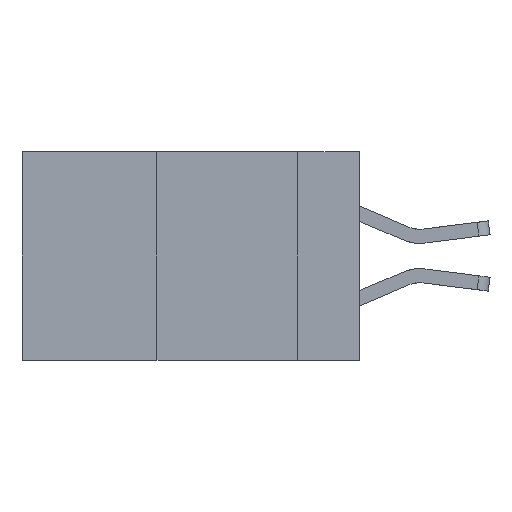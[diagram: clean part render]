
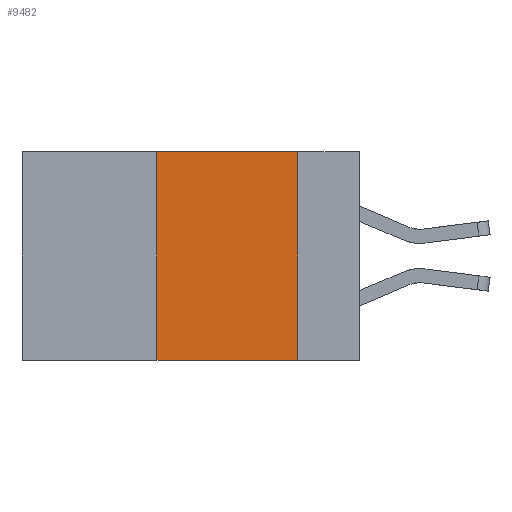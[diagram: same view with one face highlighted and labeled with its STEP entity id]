
A CAD part, left-side view. The second image highlights one B-rep face of the part: STEP entity #9482.
In plain terms, the highlighted planar face has unit normal (-1, 0, 0).
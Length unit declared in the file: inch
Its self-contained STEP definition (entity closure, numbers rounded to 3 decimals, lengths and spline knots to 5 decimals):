
#306 = EDGE_CURVE ( 'NONE', #2937, #2460, #10164, .T. ) ;
#478 = VECTOR ( 'NONE', #8379, 39.37008 ) ;
#971 = LINE ( 'NONE', #3091, #1587 ) ;
#1077 = VECTOR ( 'NONE', #9889, 39.37008 ) ;
#1249 = ORIENTED_EDGE ( 'NONE', *, *, #306, .T. ) ;
#1296 = CARTESIAN_POINT ( 'NONE',  ( 0., 0.11, -0.37 ) ) ;
#1587 = VECTOR ( 'NONE', #3090, 39.37008 ) ;
#1679 = EDGE_CURVE ( 'NONE', #2937, #5186, #971, .T. ) ;
#2460 = VERTEX_POINT ( 'NONE', #1296 ) ;
#2872 = CARTESIAN_POINT ( 'NONE',  ( 0., 0.36, -0.37 ) ) ;
#2937 = VERTEX_POINT ( 'NONE', #2872 ) ;
#2971 = CARTESIAN_POINT ( 'NONE',  ( 0., 0.36, 0. ) ) ;
#2989 = ORIENTED_EDGE ( 'NONE', *, *, #1679, .F. ) ;
#3090 = DIRECTION ( 'NONE',  ( 0., 0., 1. ) ) ;
#3091 = CARTESIAN_POINT ( 'NONE',  ( 0., 0.36, 0. ) ) ;
#3441 = EDGE_CURVE ( 'NONE', #8697, #2460, #7324, .T. ) ;
#4170 = FACE_OUTER_BOUND ( 'NONE', #7294, .T. ) ;
#4221 = VECTOR ( 'NONE', #6492, 39.37008 ) ;
#4714 = CARTESIAN_POINT ( 'NONE',  ( 0., 0.11, 0. ) ) ;
#4786 = ORIENTED_EDGE ( 'NONE', *, *, #9712, .F. ) ;
#4937 = PLANE ( 'NONE',  #10412 ) ;
#5186 = VERTEX_POINT ( 'NONE', #2971 ) ;
#5766 = CARTESIAN_POINT ( 'NONE',  ( 0., 0.6, 0. ) ) ;
#5793 = DIRECTION ( 'NONE',  ( 0., 0., -1. ) ) ;
#6481 = LINE ( 'NONE', #10576, #1077 ) ;
#6492 = DIRECTION ( 'NONE',  ( 0., -1., 0. ) ) ;
#6867 = CARTESIAN_POINT ( 'NONE',  ( 0., 0.11, 0. ) ) ;
#7124 = CARTESIAN_POINT ( 'NONE',  ( 0., 0.6, -0.37 ) ) ;
#7294 = EDGE_LOOP ( 'NONE', ( #9262, #4786, #2989, #1249 ) ) ;
#7324 = LINE ( 'NONE', #6867, #478 ) ;
#8379 = DIRECTION ( 'NONE',  ( 0., 0., -1. ) ) ;
#8697 = VERTEX_POINT ( 'NONE', #4714 ) ;
#9262 = ORIENTED_EDGE ( 'NONE', *, *, #3441, .F. ) ;
#9482 = ADVANCED_FACE ( 'NONE', ( #4170 ), #4937, .F. ) ;
#9712 = EDGE_CURVE ( 'NONE', #5186, #8697, #6481, .T. ) ;
#9889 = DIRECTION ( 'NONE',  ( 0., -1., 0. ) ) ;
#10164 = LINE ( 'NONE', #7124, #4221 ) ;
#10314 = DIRECTION ( 'NONE',  ( 1., 0., 0. ) ) ;
#10412 = AXIS2_PLACEMENT_3D ( 'NONE', #5766, #10314, #5793 ) ;
#10576 = CARTESIAN_POINT ( 'NONE',  ( 0., 0.6, 0. ) ) ;
